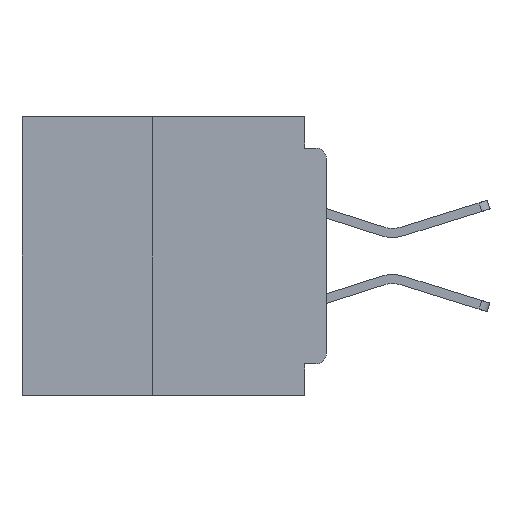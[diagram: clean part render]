
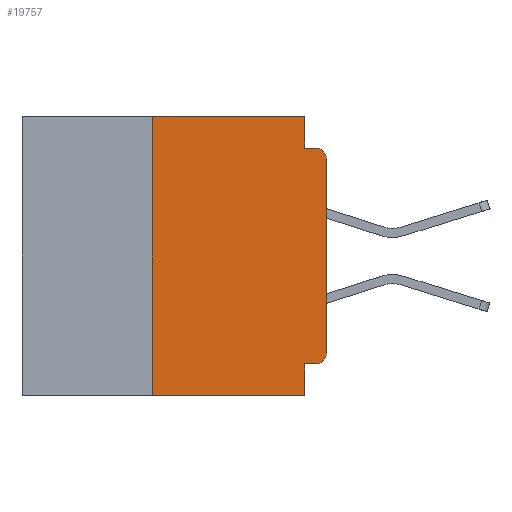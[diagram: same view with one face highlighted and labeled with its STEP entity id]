
A CAD part, left-side view. The second image highlights one B-rep face of the part: STEP entity #19757.
In plain terms, the highlighted planar face has unit normal (-1, 0, 0).
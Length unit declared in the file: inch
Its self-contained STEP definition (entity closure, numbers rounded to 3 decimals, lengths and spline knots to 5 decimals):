
#978 = LINE ( 'NONE', #4374, #24722 ) ;
#1152 = CIRCLE ( 'NONE', #38656, 0.015 ) ;
#1810 = DIRECTION ( 'NONE',  ( 0., -1., 0. ) ) ;
#2591 = VERTEX_POINT ( 'NONE', #8155 ) ;
#3827 = VECTOR ( 'NONE', #36150, 39.37008 ) ;
#4374 = CARTESIAN_POINT ( 'NONE',  ( 0., 0.437, -0.4 ) ) ;
#5108 = EDGE_CURVE ( 'NONE', #2591, #46333, #24120, .T. ) ;
#6330 = CARTESIAN_POINT ( 'NONE',  ( 0., 0.437, 0. ) ) ;
#8155 = CARTESIAN_POINT ( 'NONE',  ( 0., 0.031, -0.355 ) ) ;
#8206 = ORIENTED_EDGE ( 'NONE', *, *, #11380, .F. ) ;
#8469 = VECTOR ( 'NONE', #11458, 39.37008 ) ;
#8871 = EDGE_CURVE ( 'NONE', #23284, #46333, #978, .T. ) ;
#8961 = EDGE_CURVE ( 'NONE', #17168, #13881, #11486, .T. ) ;
#9340 = PLANE ( 'NONE',  #29369 ) ;
#9615 = CARTESIAN_POINT ( 'NONE',  ( 0., 0., -0.355 ) ) ;
#11380 = EDGE_CURVE ( 'NONE', #13881, #33909, #20384, .T. ) ;
#11458 = DIRECTION ( 'NONE',  ( 0., -1., 0. ) ) ;
#11486 = LINE ( 'NONE', #31606, #19237 ) ;
#11487 = VERTEX_POINT ( 'NONE', #25455 ) ;
#12465 = CARTESIAN_POINT ( 'NONE',  ( 0., 0.015, -0.34 ) ) ;
#13809 = AXIS2_PLACEMENT_3D ( 'NONE', #12465, #43378, #16992 ) ;
#13881 = VERTEX_POINT ( 'NONE', #18513 ) ;
#16667 = EDGE_CURVE ( 'NONE', #45804, #11487, #52268, .T. ) ;
#16992 = DIRECTION ( 'NONE',  ( 0., 0., -1. ) ) ;
#17125 = VECTOR ( 'NONE', #31494, 39.37008 ) ;
#17168 = VERTEX_POINT ( 'NONE', #44359 ) ;
#17800 = LINE ( 'NONE', #27617, #50131 ) ;
#17959 = VERTEX_POINT ( 'NONE', #18689 ) ;
#18345 = CARTESIAN_POINT ( 'NONE',  ( 0., 0.031, -0.4 ) ) ;
#18398 = CARTESIAN_POINT ( 'NONE',  ( 0., 0.437, 0. ) ) ;
#18513 = CARTESIAN_POINT ( 'NONE',  ( 0., 0.031, -0.045 ) ) ;
#18689 = CARTESIAN_POINT ( 'NONE',  ( 0., 0.015, -0.355 ) ) ;
#19136 = EDGE_LOOP ( 'NONE', ( #29333, #46841, #8206, #25110, #55980, #20033, #35059, #35073, #28423, #29803 ) ) ;
#19237 = VECTOR ( 'NONE', #53568, 39.37008 ) ;
#19638 = CIRCLE ( 'NONE', #13809, 0.015 ) ;
#19757 = ADVANCED_FACE ( 'NONE', ( #51428 ), #9340, .F. ) ;
#20033 = ORIENTED_EDGE ( 'NONE', *, *, #26882, .F. ) ;
#20384 = LINE ( 'NONE', #46655, #8469 ) ;
#21804 = CARTESIAN_POINT ( 'NONE',  ( 0., 0.031, -0.4 ) ) ;
#22816 = DIRECTION ( 'NONE',  ( 0., 0., -1. ) ) ;
#23190 = DIRECTION ( 'NONE',  ( 0., 0., 1. ) ) ;
#23284 = VERTEX_POINT ( 'NONE', #25637 ) ;
#24120 = LINE ( 'NONE', #21804, #33067 ) ;
#24722 = VECTOR ( 'NONE', #35481, 39.37008 ) ;
#24862 = DIRECTION ( 'NONE',  ( -1., 0., 0. ) ) ;
#25110 = ORIENTED_EDGE ( 'NONE', *, *, #8961, .F. ) ;
#25455 = CARTESIAN_POINT ( 'NONE',  ( 0., 0., -0.06 ) ) ;
#25637 = CARTESIAN_POINT ( 'NONE',  ( 0., 0.25, -0.4 ) ) ;
#26758 = CARTESIAN_POINT ( 'NONE',  ( 0., 0.015, -0.045 ) ) ;
#26882 = EDGE_CURVE ( 'NONE', #23284, #38116, #17800, .T. ) ;
#27617 = CARTESIAN_POINT ( 'NONE',  ( 0., 0.25, -0.4 ) ) ;
#28423 = ORIENTED_EDGE ( 'NONE', *, *, #46985, .F. ) ;
#28773 = EDGE_CURVE ( 'NONE', #17959, #45804, #19638, .T. ) ;
#29333 = ORIENTED_EDGE ( 'NONE', *, *, #16667, .T. ) ;
#29369 = AXIS2_PLACEMENT_3D ( 'NONE', #18398, #49157, #22816 ) ;
#29803 = ORIENTED_EDGE ( 'NONE', *, *, #28773, .T. ) ;
#31494 = DIRECTION ( 'NONE',  ( 0., 0., 1. ) ) ;
#31606 = CARTESIAN_POINT ( 'NONE',  ( 0., 0.031, 0. ) ) ;
#33067 = VECTOR ( 'NONE', #43765, 39.37008 ) ;
#33550 = EDGE_CURVE ( 'NONE', #38116, #17168, #53310, .T. ) ;
#33909 = VERTEX_POINT ( 'NONE', #26758 ) ;
#34761 = EDGE_CURVE ( 'NONE', #11487, #33909, #1152, .T. ) ;
#35059 = ORIENTED_EDGE ( 'NONE', *, *, #8871, .T. ) ;
#35073 = ORIENTED_EDGE ( 'NONE', *, *, #5108, .F. ) ;
#35481 = DIRECTION ( 'NONE',  ( 0., -1., 0. ) ) ;
#36150 = DIRECTION ( 'NONE',  ( 0., 1., 0. ) ) ;
#38116 = VERTEX_POINT ( 'NONE', #40069 ) ;
#38656 = AXIS2_PLACEMENT_3D ( 'NONE', #51225, #24862, #55673 ) ;
#40069 = CARTESIAN_POINT ( 'NONE',  ( 0., 0.25, 0. ) ) ;
#41583 = VECTOR ( 'NONE', #1810, 39.37008 ) ;
#43378 = DIRECTION ( 'NONE',  ( -1., 0., 0. ) ) ;
#43765 = DIRECTION ( 'NONE',  ( 0., 0., -1. ) ) ;
#44359 = CARTESIAN_POINT ( 'NONE',  ( 0., 0.031, 0. ) ) ;
#45804 = VERTEX_POINT ( 'NONE', #50304 ) ;
#46333 = VERTEX_POINT ( 'NONE', #18345 ) ;
#46655 = CARTESIAN_POINT ( 'NONE',  ( 0., 0., -0.045 ) ) ;
#46841 = ORIENTED_EDGE ( 'NONE', *, *, #34761, .T. ) ;
#46985 = EDGE_CURVE ( 'NONE', #17959, #2591, #49575, .T. ) ;
#49157 = DIRECTION ( 'NONE',  ( 1., 0., 0. ) ) ;
#49575 = LINE ( 'NONE', #9615, #3827 ) ;
#50131 = VECTOR ( 'NONE', #23190, 39.37008 ) ;
#50304 = CARTESIAN_POINT ( 'NONE',  ( 0., 0., -0.34 ) ) ;
#51225 = CARTESIAN_POINT ( 'NONE',  ( 0., 0.015, -0.06 ) ) ;
#51428 = FACE_OUTER_BOUND ( 'NONE', #19136, .T. ) ;
#52268 = LINE ( 'NONE', #53452, #17125 ) ;
#53310 = LINE ( 'NONE', #6330, #41583 ) ;
#53452 = CARTESIAN_POINT ( 'NONE',  ( 0., 0., 0. ) ) ;
#53568 = DIRECTION ( 'NONE',  ( 0., 0., -1. ) ) ;
#55673 = DIRECTION ( 'NONE',  ( 0., 0., -1. ) ) ;
#55980 = ORIENTED_EDGE ( 'NONE', *, *, #33550, .F. ) ;
